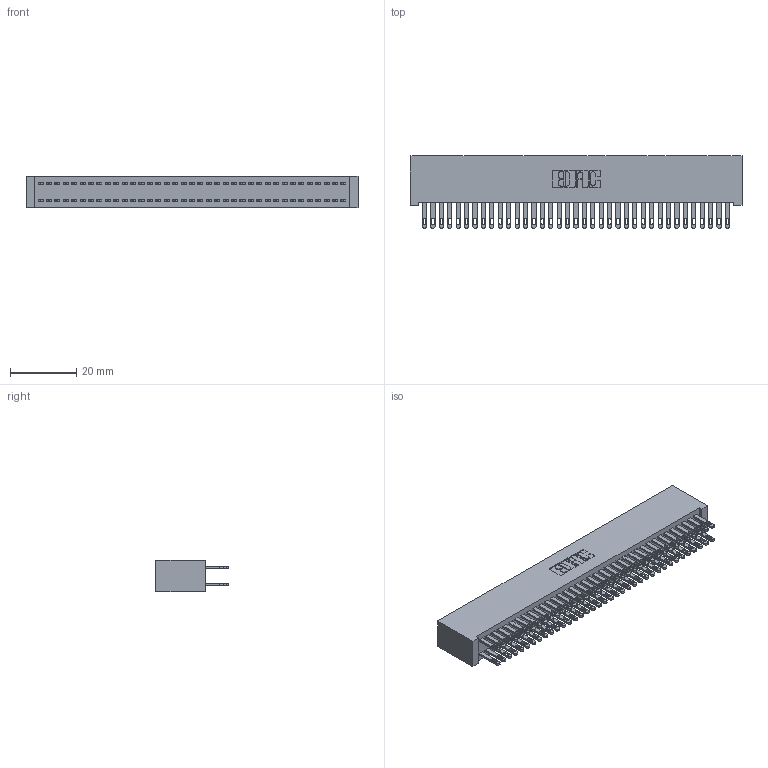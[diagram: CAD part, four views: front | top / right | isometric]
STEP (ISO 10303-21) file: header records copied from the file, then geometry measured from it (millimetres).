
FILE_DESCRIPTION (( 'STEP AP203' ), '1' );
FILE_NAME ('892-074-500-201.STEP', '2020-09-21T19:50:11', ( '' ), ( '' ), 'SwSTEP 2.0', 'SolidWorks 2020', '' );
FILE_SCHEMA (( 'CONFIG_CONTROL_DESIGN' ));
Length unit declared in the file: inch
Products named in the file (3): 892-074-500-201; 842 Part_Lugless; 345-292-001_345-293-100
Assembly tree (75 placements, depth 2):
  892-074-500-201
    842 Part_Lugless
    345-292-001_345-293-100  x74
Bounding box: 100.23 x 21.85 x 9.4 mm (x, y, z)
Volume: 9647.5 mm3; surface area: 16735.2 mm2
Topology: 75 solids, 75 shells, 3654 faces, 11153 edges, 7434 vertices
Faces by surface type: plane 2282, cylinder 1372
Entity records: 23971 total; most frequent: CARTESIAN_POINT 3974, ORIENTED_EDGE 3910, DIRECTION 3399, EDGE_CURVE 1955, LINE 1831, VECTOR 1831, VERTEX_POINT 1302, AXIS2_PLACEMENT_3D 784
